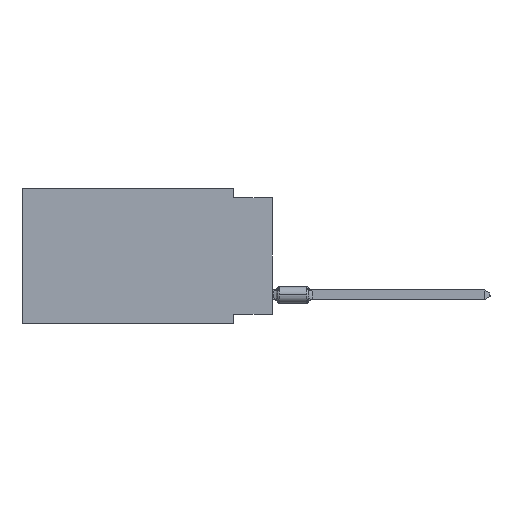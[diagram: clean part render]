
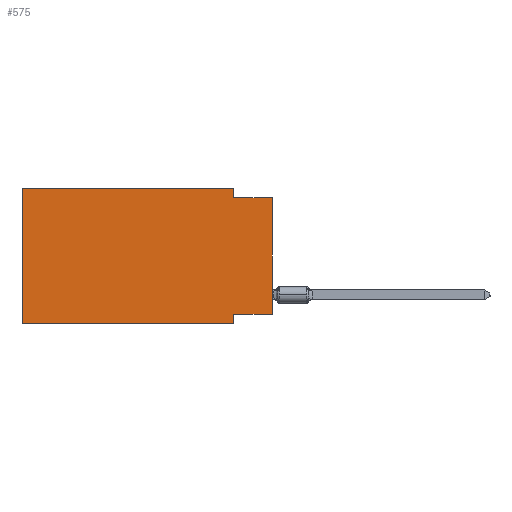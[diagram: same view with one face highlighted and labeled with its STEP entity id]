
A CAD part, left-side view. The second image highlights one B-rep face of the part: STEP entity #575.
In plain terms, the highlighted planar face has unit normal (-1, 0, 0).
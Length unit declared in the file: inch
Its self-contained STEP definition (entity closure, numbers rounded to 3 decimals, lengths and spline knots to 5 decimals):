
#575 = ADVANCED_FACE ( 'NONE', ( #49812 ), #25496, .F. ) ;
#608 = ORIENTED_EDGE ( 'NONE', *, *, #26396, .T. ) ;
#1749 = EDGE_CURVE ( 'NONE', #25063, #35545, #15367, .T. ) ;
#2484 = ORIENTED_EDGE ( 'NONE', *, *, #1749, .F. ) ;
#2639 = LINE ( 'NONE', #11608, #33855 ) ;
#2698 = VERTEX_POINT ( 'NONE', #21836 ) ;
#4300 = LINE ( 'NONE', #34070, #5417 ) ;
#5417 = VECTOR ( 'NONE', #53608, 39.37008 ) ;
#5748 = ORIENTED_EDGE ( 'NONE', *, *, #59747, .F. ) ;
#9047 = CARTESIAN_POINT ( 'NONE',  ( 0., 0., -0.025 ) ) ;
#10250 = DIRECTION ( 'NONE',  ( 0., -1., 0. ) ) ;
#10416 = EDGE_CURVE ( 'NONE', #36727, #35545, #10430, .T. ) ;
#10430 = LINE ( 'NONE', #11681, #37520 ) ;
#11608 = CARTESIAN_POINT ( 'NONE',  ( 0., 0., -0.325 ) ) ;
#11681 = CARTESIAN_POINT ( 'NONE',  ( 0., 0., 0. ) ) ;
#12343 = DIRECTION ( 'NONE',  ( 0., 0., -1. ) ) ;
#12777 = CARTESIAN_POINT ( 'NONE',  ( 0., 0.645, 0. ) ) ;
#14407 = VECTOR ( 'NONE', #22376, 39.37008 ) ;
#15367 = LINE ( 'NONE', #34888, #26920 ) ;
#19991 = VERTEX_POINT ( 'NONE', #20516 ) ;
#20041 = EDGE_CURVE ( 'NONE', #24418, #2698, #25026, .T. ) ;
#20207 = DIRECTION ( 'NONE',  ( 0., -1., 0. ) ) ;
#20516 = CARTESIAN_POINT ( 'NONE',  ( 0., 0.1, -0.325 ) ) ;
#20713 = CARTESIAN_POINT ( 'NONE',  ( 0., 0.645, 0. ) ) ;
#21007 = DIRECTION ( 'NONE',  ( 1., 0., 0. ) ) ;
#21836 = CARTESIAN_POINT ( 'NONE',  ( 0., 0.1, 0. ) ) ;
#22145 = DIRECTION ( 'NONE',  ( 0., 1., 0. ) ) ;
#22376 = DIRECTION ( 'NONE',  ( 0., 0., 1. ) ) ;
#24418 = VERTEX_POINT ( 'NONE', #63012 ) ;
#24973 = EDGE_CURVE ( 'NONE', #36727, #19991, #2639, .T. ) ;
#25026 = LINE ( 'NONE', #59879, #46218 ) ;
#25063 = VERTEX_POINT ( 'NONE', #48390 ) ;
#25496 = PLANE ( 'NONE',  #54669 ) ;
#26396 = EDGE_CURVE ( 'NONE', #56847, #57766, #4300, .T. ) ;
#26751 = DIRECTION ( 'NONE',  ( 0., 0., -1. ) ) ;
#26920 = VECTOR ( 'NONE', #10250, 39.37008 ) ;
#28998 = ORIENTED_EDGE ( 'NONE', *, *, #54157, .F. ) ;
#29312 = EDGE_LOOP ( 'NONE', ( #54384, #2484, #52747, #48450, #5748, #608, #28998, #33108 ) ) ;
#33108 = ORIENTED_EDGE ( 'NONE', *, *, #24973, .F. ) ;
#33855 = VECTOR ( 'NONE', #22145, 39.37008 ) ;
#34070 = CARTESIAN_POINT ( 'NONE',  ( 0., 0.645, -0.35 ) ) ;
#34888 = CARTESIAN_POINT ( 'NONE',  ( 0., 0., -0.025 ) ) ;
#35545 = VERTEX_POINT ( 'NONE', #9047 ) ;
#36727 = VERTEX_POINT ( 'NONE', #59764 ) ;
#37520 = VECTOR ( 'NONE', #54893, 39.37008 ) ;
#38615 = CARTESIAN_POINT ( 'NONE',  ( 0., 0.645, -0.35 ) ) ;
#40506 = DIRECTION ( 'NONE',  ( 0., 0., -1. ) ) ;
#41779 = CARTESIAN_POINT ( 'NONE',  ( 0., 0.1, 0. ) ) ;
#45755 = LINE ( 'NONE', #12777, #14407 ) ;
#46218 = VECTOR ( 'NONE', #20207, 39.37008 ) ;
#48390 = CARTESIAN_POINT ( 'NONE',  ( 0., 0.1, -0.025 ) ) ;
#48450 = ORIENTED_EDGE ( 'NONE', *, *, #20041, .F. ) ;
#49812 = FACE_OUTER_BOUND ( 'NONE', #29312, .T. ) ;
#51042 = VECTOR ( 'NONE', #12343, 39.37008 ) ;
#51077 = LINE ( 'NONE', #41779, #58187 ) ;
#52747 = ORIENTED_EDGE ( 'NONE', *, *, #54053, .F. ) ;
#53608 = DIRECTION ( 'NONE',  ( 0., -1., 0. ) ) ;
#54053 = EDGE_CURVE ( 'NONE', #2698, #25063, #51077, .T. ) ;
#54157 = EDGE_CURVE ( 'NONE', #19991, #57766, #61019, .T. ) ;
#54384 = ORIENTED_EDGE ( 'NONE', *, *, #10416, .T. ) ;
#54669 = AXIS2_PLACEMENT_3D ( 'NONE', #20713, #21007, #40506 ) ;
#54893 = DIRECTION ( 'NONE',  ( 0., 0., 1. ) ) ;
#56210 = CARTESIAN_POINT ( 'NONE',  ( 0., 0.1, -0.35 ) ) ;
#56847 = VERTEX_POINT ( 'NONE', #38615 ) ;
#57766 = VERTEX_POINT ( 'NONE', #62109 ) ;
#58187 = VECTOR ( 'NONE', #26751, 39.37008 ) ;
#59747 = EDGE_CURVE ( 'NONE', #56847, #24418, #45755, .T. ) ;
#59764 = CARTESIAN_POINT ( 'NONE',  ( 0., 0., -0.325 ) ) ;
#59879 = CARTESIAN_POINT ( 'NONE',  ( 0., 0.645, 0. ) ) ;
#61019 = LINE ( 'NONE', #56210, #51042 ) ;
#62109 = CARTESIAN_POINT ( 'NONE',  ( 0., 0.1, -0.35 ) ) ;
#63012 = CARTESIAN_POINT ( 'NONE',  ( 0., 0.645, 0. ) ) ;
